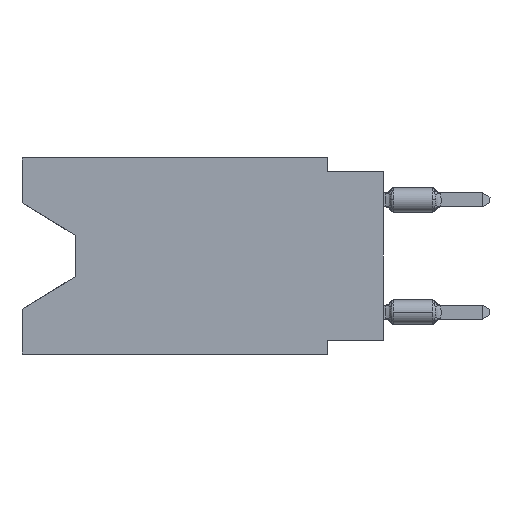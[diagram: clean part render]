
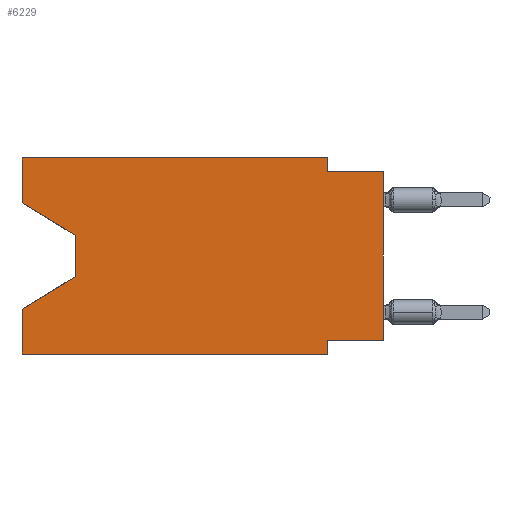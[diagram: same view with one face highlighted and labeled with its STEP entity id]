
A CAD part, left-side view. The second image highlights one B-rep face of the part: STEP entity #6229.
In plain terms, the highlighted planar face has unit normal (-1, 0, 0).
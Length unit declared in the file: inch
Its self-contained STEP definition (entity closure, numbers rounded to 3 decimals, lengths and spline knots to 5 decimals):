
#396 = VERTEX_POINT ( 'NONE', #4516 ) ;
#709 = VECTOR ( 'NONE', #6510, 39.37008 ) ;
#818 = CARTESIAN_POINT ( 'NONE',  ( 0., 0.55, -0.138 ) ) ;
#1182 = VECTOR ( 'NONE', #14372, 39.37008 ) ;
#1621 = CARTESIAN_POINT ( 'NONE',  ( 0., 0.645, -0.08025 ) ) ;
#1953 = ORIENTED_EDGE ( 'NONE', *, *, #12278, .T. ) ;
#2202 = ORIENTED_EDGE ( 'NONE', *, *, #18135, .T. ) ;
#2292 = LINE ( 'NONE', #9403, #18919 ) ;
#2395 = ORIENTED_EDGE ( 'NONE', *, *, #2575, .T. ) ;
#2422 = ORIENTED_EDGE ( 'NONE', *, *, #7601, .T. ) ;
#2553 = DIRECTION ( 'NONE',  ( 0., 1., 0. ) ) ;
#2575 = EDGE_CURVE ( 'NONE', #16584, #12169, #4105, .T. ) ;
#3123 = CARTESIAN_POINT ( 'NONE',  ( 0., 0.645, 0. ) ) ;
#3210 = CARTESIAN_POINT ( 'NONE',  ( 0., 0.645, -0.26975 ) ) ;
#3645 = LINE ( 'NONE', #15903, #1182 ) ;
#4095 = CARTESIAN_POINT ( 'NONE',  ( 0., 0., -0.325 ) ) ;
#4105 = LINE ( 'NONE', #4319, #20472 ) ;
#4319 = CARTESIAN_POINT ( 'NONE',  ( 0., 0.55, -0.138 ) ) ;
#4443 = CARTESIAN_POINT ( 'NONE',  ( 0., 0.55, -0.212 ) ) ;
#4516 = CARTESIAN_POINT ( 'NONE',  ( 0., 0.1, -0.35 ) ) ;
#4594 = CARTESIAN_POINT ( 'NONE',  ( 0., 0.645, 0. ) ) ;
#4602 = CARTESIAN_POINT ( 'NONE',  ( 0., 0., -0.025 ) ) ;
#4712 = DIRECTION ( 'NONE',  ( 0., 0., -1. ) ) ;
#5206 = VERTEX_POINT ( 'NONE', #16784 ) ;
#5470 = LINE ( 'NONE', #1621, #10969 ) ;
#5606 = CARTESIAN_POINT ( 'NONE',  ( 0., 0., -0.025 ) ) ;
#5894 = ORIENTED_EDGE ( 'NONE', *, *, #10534, .F. ) ;
#6012 = VERTEX_POINT ( 'NONE', #11778 ) ;
#6229 = ADVANCED_FACE ( 'NONE', ( #6324 ), #13456, .F. ) ;
#6261 = CARTESIAN_POINT ( 'NONE',  ( 0., 0.645, 0. ) ) ;
#6324 = FACE_OUTER_BOUND ( 'NONE', #17201, .T. ) ;
#6396 = CARTESIAN_POINT ( 'NONE',  ( 0., 0., -0.325 ) ) ;
#6510 = DIRECTION ( 'NONE',  ( 0., 0., -1. ) ) ;
#6579 = ORIENTED_EDGE ( 'NONE', *, *, #18368, .F. ) ;
#6580 = CARTESIAN_POINT ( 'NONE',  ( 0., 0.1, -0.325 ) ) ;
#7024 = VECTOR ( 'NONE', #2553, 39.37008 ) ;
#7255 = LINE ( 'NONE', #10420, #7873 ) ;
#7545 = EDGE_CURVE ( 'NONE', #6012, #22012, #3645, .T. ) ;
#7601 = EDGE_CURVE ( 'NONE', #8822, #10443, #7255, .T. ) ;
#7873 = VECTOR ( 'NONE', #12292, 39.37008 ) ;
#7974 = LINE ( 'NONE', #8096, #9699 ) ;
#8096 = CARTESIAN_POINT ( 'NONE',  ( 0., 0.645, 0. ) ) ;
#8723 = CARTESIAN_POINT ( 'NONE',  ( 0., 0.1, -0.025 ) ) ;
#8739 = LINE ( 'NONE', #15856, #709 ) ;
#8822 = VERTEX_POINT ( 'NONE', #4095 ) ;
#8877 = AXIS2_PLACEMENT_3D ( 'NONE', #4594, #13569, #4712 ) ;
#8985 = LINE ( 'NONE', #16106, #16023 ) ;
#9403 = CARTESIAN_POINT ( 'NONE',  ( 0., 0.645, 0. ) ) ;
#9699 = VECTOR ( 'NONE', #22394, 39.37008 ) ;
#9837 = EDGE_CURVE ( 'NONE', #22012, #10443, #20619, .T. ) ;
#10158 = CARTESIAN_POINT ( 'NONE',  ( 0., 0.55, -0.212 ) ) ;
#10353 = DIRECTION ( 'NONE',  ( 0., -1., 0. ) ) ;
#10420 = CARTESIAN_POINT ( 'NONE',  ( 0., 0., 0. ) ) ;
#10443 = VERTEX_POINT ( 'NONE', #5606 ) ;
#10534 = EDGE_CURVE ( 'NONE', #8822, #22384, #20792, .T. ) ;
#10618 = DIRECTION ( 'NONE',  ( 0., -1., 0. ) ) ;
#10969 = VECTOR ( 'NONE', #17989, 39.37008 ) ;
#11215 = DIRECTION ( 'NONE',  ( 0., 0., -1. ) ) ;
#11553 = DIRECTION ( 'NONE',  ( 0., 0.855, -0.519 ) ) ;
#11778 = CARTESIAN_POINT ( 'NONE',  ( 0., 0.1, 0. ) ) ;
#12101 = EDGE_CURVE ( 'NONE', #12169, #13000, #15166, .T. ) ;
#12169 = VERTEX_POINT ( 'NONE', #10158 ) ;
#12278 = EDGE_CURVE ( 'NONE', #17806, #396, #8985, .T. ) ;
#12292 = DIRECTION ( 'NONE',  ( 0., 0., 1. ) ) ;
#12853 = VECTOR ( 'NONE', #10353, 39.37008 ) ;
#12888 = EDGE_CURVE ( 'NONE', #17806, #13000, #7974, .T. ) ;
#13000 = VERTEX_POINT ( 'NONE', #3210 ) ;
#13456 = PLANE ( 'NONE',  #8877 ) ;
#13569 = DIRECTION ( 'NONE',  ( 1., 0., 0. ) ) ;
#14372 = DIRECTION ( 'NONE',  ( 0., 0., -1. ) ) ;
#14879 = ORIENTED_EDGE ( 'NONE', *, *, #22189, .F. ) ;
#15166 = LINE ( 'NONE', #4443, #15262 ) ;
#15262 = VECTOR ( 'NONE', #11553, 39.37008 ) ;
#15856 = CARTESIAN_POINT ( 'NONE',  ( 0., 0.1, -0.35 ) ) ;
#15903 = CARTESIAN_POINT ( 'NONE',  ( 0., 0.1, 0. ) ) ;
#16023 = VECTOR ( 'NONE', #10618, 39.37008 ) ;
#16106 = CARTESIAN_POINT ( 'NONE',  ( 0., 0.645, -0.35 ) ) ;
#16584 = VERTEX_POINT ( 'NONE', #818 ) ;
#16784 = CARTESIAN_POINT ( 'NONE',  ( 0., 0.645, -0.08025 ) ) ;
#17094 = DIRECTION ( 'NONE',  ( 0., -1., 0. ) ) ;
#17201 = EDGE_LOOP ( 'NONE', ( #2202, #2395, #18985, #19650, #1953, #19025, #5894, #2422, #18832, #18035, #6579, #14879 ) ) ;
#17806 = VERTEX_POINT ( 'NONE', #20575 ) ;
#17989 = DIRECTION ( 'NONE',  ( 0., -0.855, -0.519 ) ) ;
#18035 = ORIENTED_EDGE ( 'NONE', *, *, #7545, .F. ) ;
#18135 = EDGE_CURVE ( 'NONE', #5206, #16584, #5470, .T. ) ;
#18360 = VERTEX_POINT ( 'NONE', #6261 ) ;
#18368 = EDGE_CURVE ( 'NONE', #18360, #6012, #19136, .T. ) ;
#18832 = ORIENTED_EDGE ( 'NONE', *, *, #9837, .F. ) ;
#18919 = VECTOR ( 'NONE', #21586, 39.37008 ) ;
#18985 = ORIENTED_EDGE ( 'NONE', *, *, #12101, .T. ) ;
#19025 = ORIENTED_EDGE ( 'NONE', *, *, #19760, .F. ) ;
#19136 = LINE ( 'NONE', #3123, #12853 ) ;
#19650 = ORIENTED_EDGE ( 'NONE', *, *, #12888, .F. ) ;
#19760 = EDGE_CURVE ( 'NONE', #22384, #396, #8739, .T. ) ;
#20472 = VECTOR ( 'NONE', #11215, 39.37008 ) ;
#20575 = CARTESIAN_POINT ( 'NONE',  ( 0., 0.645, -0.35 ) ) ;
#20619 = LINE ( 'NONE', #4602, #21578 ) ;
#20792 = LINE ( 'NONE', #6396, #7024 ) ;
#21578 = VECTOR ( 'NONE', #17094, 39.37008 ) ;
#21586 = DIRECTION ( 'NONE',  ( 0., 0., 1. ) ) ;
#22012 = VERTEX_POINT ( 'NONE', #8723 ) ;
#22189 = EDGE_CURVE ( 'NONE', #5206, #18360, #2292, .T. ) ;
#22384 = VERTEX_POINT ( 'NONE', #6580 ) ;
#22394 = DIRECTION ( 'NONE',  ( 0., 0., 1. ) ) ;
